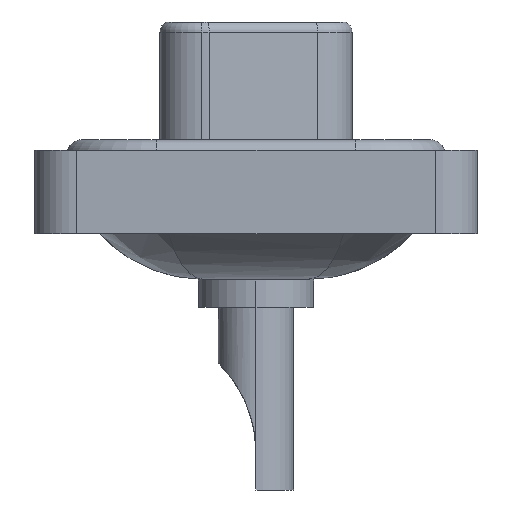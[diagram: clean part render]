
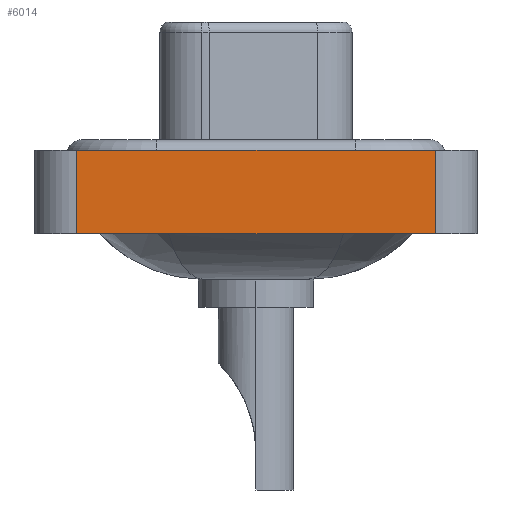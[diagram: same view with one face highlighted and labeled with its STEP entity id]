
A CAD part, left-side view. The second image highlights one B-rep face of the part: STEP entity #6014.
In plain terms, the highlighted planar face has unit normal (-1, 0, 0).
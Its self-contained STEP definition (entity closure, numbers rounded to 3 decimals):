
#1285 = VERTEX_POINT ( 'NONE', #1841 ) ;
#1841 = CARTESIAN_POINT ( 'NONE',  ( -7.25, -8.55, -3.6 ) ) ;
#2896 = LINE ( 'NONE', #14221, #11717 ) ;
#4496 = CARTESIAN_POINT ( 'NONE',  ( -7.25, -8.55, -3.6 ) ) ;
#5480 = VERTEX_POINT ( 'NONE', #17289 ) ;
#5750 = EDGE_LOOP ( 'NONE', ( #11937, #17163, #16560, #18047 ) ) ;
#6014 = ADVANCED_FACE ( 'NONE', ( #10797 ), #6496, .T. ) ;
#6413 = CARTESIAN_POINT ( 'NONE',  ( -7.25, -8.55, -3.6 ) ) ;
#6496 = PLANE ( 'NONE',  #7889 ) ;
#6593 = DIRECTION ( 'NONE',  ( -1., 0., 0. ) ) ;
#6623 = DIRECTION ( 'NONE',  ( 0., 0., 1. ) ) ;
#7889 = AXIS2_PLACEMENT_3D ( 'NONE', #6413, #6593, #7988 ) ;
#7988 = DIRECTION ( 'NONE',  ( 0., 0., 1. ) ) ;
#8299 = CARTESIAN_POINT ( 'NONE',  ( -7.25, 8.55, -3.6 ) ) ;
#8748 = EDGE_CURVE ( 'NONE', #17794, #12660, #17926, .T. ) ;
#9513 = CARTESIAN_POINT ( 'NONE',  ( -7.25, -8.55, -3.6 ) ) ;
#10310 = CARTESIAN_POINT ( 'NONE',  ( -7.25, 8.55, 0.4 ) ) ;
#10797 = FACE_OUTER_BOUND ( 'NONE', #5750, .T. ) ;
#11503 = LINE ( 'NONE', #4496, #17642 ) ;
#11510 = DIRECTION ( 'NONE',  ( 0., -1., 0. ) ) ;
#11717 = VECTOR ( 'NONE', #11510, 1000. ) ;
#11784 = DIRECTION ( 'NONE',  ( 0., -1., 0. ) ) ;
#11937 = ORIENTED_EDGE ( 'NONE', *, *, #15366, .T. ) ;
#12267 = VECTOR ( 'NONE', #6623, 1000. ) ;
#12660 = VERTEX_POINT ( 'NONE', #10310 ) ;
#13209 = EDGE_CURVE ( 'NONE', #17794, #1285, #11503, .T. ) ;
#13499 = CARTESIAN_POINT ( 'NONE',  ( -7.25, 8.55, -3.6 ) ) ;
#14221 = CARTESIAN_POINT ( 'NONE',  ( -7.25, -8.55, 0.4 ) ) ;
#14569 = VECTOR ( 'NONE', #15230, 1000. ) ;
#15131 = EDGE_CURVE ( 'NONE', #12660, #5480, #2896, .T. ) ;
#15230 = DIRECTION ( 'NONE',  ( 0., 0., 1. ) ) ;
#15366 = EDGE_CURVE ( 'NONE', #1285, #5480, #16288, .T. ) ;
#16288 = LINE ( 'NONE', #9513, #14569 ) ;
#16560 = ORIENTED_EDGE ( 'NONE', *, *, #8748, .F. ) ;
#17163 = ORIENTED_EDGE ( 'NONE', *, *, #15131, .F. ) ;
#17289 = CARTESIAN_POINT ( 'NONE',  ( -7.25, -8.55, 0.4 ) ) ;
#17642 = VECTOR ( 'NONE', #11784, 1000. ) ;
#17794 = VERTEX_POINT ( 'NONE', #13499 ) ;
#17926 = LINE ( 'NONE', #8299, #12267 ) ;
#18047 = ORIENTED_EDGE ( 'NONE', *, *, #13209, .T. ) ;
